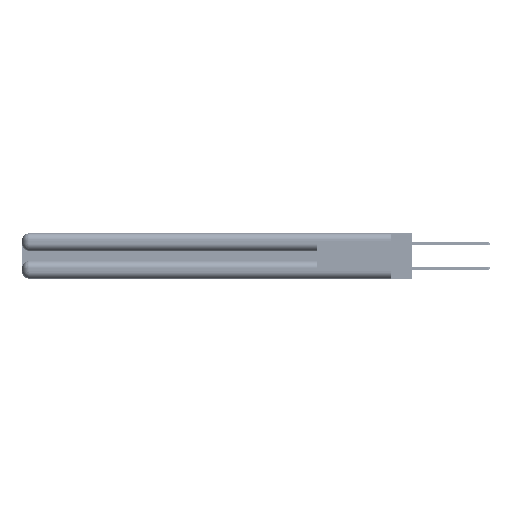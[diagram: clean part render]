
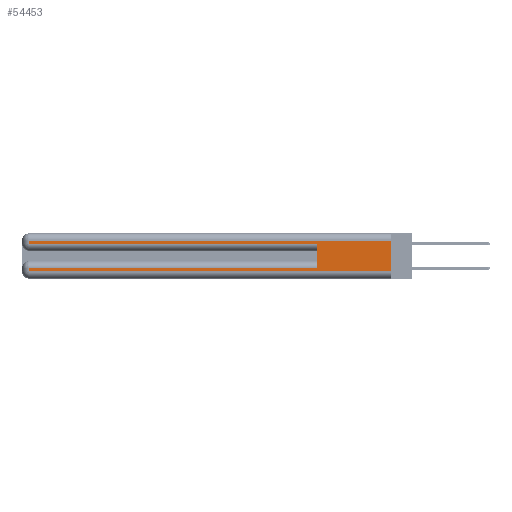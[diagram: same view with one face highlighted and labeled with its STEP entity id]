
A CAD part, left-side view. The second image highlights one B-rep face of the part: STEP entity #54453.
In plain terms, the highlighted planar face has unit normal (-1, 0, 0).
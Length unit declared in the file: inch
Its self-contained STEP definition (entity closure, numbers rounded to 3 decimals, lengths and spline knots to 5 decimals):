
#47 = ORIENTED_EDGE ( 'NONE', *, *, #4974, .T. ) ;
#947 = ORIENTED_EDGE ( 'NONE', *, *, #12364, .T. ) ;
#1749 = CARTESIAN_POINT ( 'NONE',  ( 0., 0.6, 0.285 ) ) ;
#1974 = VECTOR ( 'NONE', #44980, 39.37008 ) ;
#4145 = VECTOR ( 'NONE', #28373, 39.37008 ) ;
#4375 = DIRECTION ( 'NONE',  ( 0., 1., 0. ) ) ;
#4974 = EDGE_CURVE ( 'NONE', #36044, #13295, #21427, .T. ) ;
#5065 = VECTOR ( 'NONE', #9679, 39.37008 ) ;
#5963 = CARTESIAN_POINT ( 'NONE',  ( 0., 2.94, 0.085 ) ) ;
#7290 = ORIENTED_EDGE ( 'NONE', *, *, #31263, .F. ) ;
#8064 = VERTEX_POINT ( 'NONE', #47664 ) ;
#8731 = DIRECTION ( 'NONE',  ( 0., 0., -1. ) ) ;
#9679 = DIRECTION ( 'NONE',  ( 0., 0., -1. ) ) ;
#10702 = CARTESIAN_POINT ( 'NONE',  ( 0., 2.94, 0.285 ) ) ;
#10951 = DIRECTION ( 'NONE',  ( 0., -1., 0. ) ) ;
#12364 = EDGE_CURVE ( 'NONE', #24247, #8064, #53067, .T. ) ;
#13295 = VERTEX_POINT ( 'NONE', #27167 ) ;
#13397 = VERTEX_POINT ( 'NONE', #1749 ) ;
#13439 = EDGE_CURVE ( 'NONE', #8064, #55235, #55039, .T. ) ;
#14025 = CARTESIAN_POINT ( 'NONE',  ( 0., 0., 0.37 ) ) ;
#14072 = FACE_OUTER_BOUND ( 'NONE', #21732, .T. ) ;
#14508 = EDGE_CURVE ( 'NONE', #13295, #37177, #39589, .T. ) ;
#16024 = CARTESIAN_POINT ( 'NONE',  ( 0., 0., 0.37 ) ) ;
#16612 = EDGE_CURVE ( 'NONE', #40593, #13397, #27222, .T. ) ;
#17777 = EDGE_CURVE ( 'NONE', #37177, #13397, #35202, .T. ) ;
#18070 = VECTOR ( 'NONE', #20364, 39.37008 ) ;
#18396 = DIRECTION ( 'NONE',  ( 0., 0., -1. ) ) ;
#20364 = DIRECTION ( 'NONE',  ( 0., 0., -1. ) ) ;
#21288 = CARTESIAN_POINT ( 'NONE',  ( 0., 0.6, 0.085 ) ) ;
#21427 = LINE ( 'NONE', #52797, #44275 ) ;
#21708 = CARTESIAN_POINT ( 'NONE',  ( 0., 0., 0.085 ) ) ;
#21732 = EDGE_LOOP ( 'NONE', ( #7290, #47, #43941, #53854, #28434, #35657, #947, #35711 ) ) ;
#22550 = PLANE ( 'NONE',  #35473 ) ;
#22808 = DIRECTION ( 'NONE',  ( 0., 1., 0. ) ) ;
#24247 = VERTEX_POINT ( 'NONE', #5963 ) ;
#27167 = CARTESIAN_POINT ( 'NONE',  ( 0., 2.94, 0.31 ) ) ;
#27222 = LINE ( 'NONE', #41170, #4145 ) ;
#28373 = DIRECTION ( 'NONE',  ( 0., 0., 1. ) ) ;
#28434 = ORIENTED_EDGE ( 'NONE', *, *, #16612, .F. ) ;
#31263 = EDGE_CURVE ( 'NONE', #36044, #55235, #52309, .T. ) ;
#31639 = VECTOR ( 'NONE', #8731, 39.37008 ) ;
#35202 = LINE ( 'NONE', #44792, #1974 ) ;
#35473 = AXIS2_PLACEMENT_3D ( 'NONE', #14025, #44140, #18396 ) ;
#35657 = ORIENTED_EDGE ( 'NONE', *, *, #41909, .T. ) ;
#35711 = ORIENTED_EDGE ( 'NONE', *, *, #13439, .T. ) ;
#36044 = VERTEX_POINT ( 'NONE', #37216 ) ;
#37177 = VERTEX_POINT ( 'NONE', #10702 ) ;
#37216 = CARTESIAN_POINT ( 'NONE',  ( 0., 0., 0.31 ) ) ;
#39589 = LINE ( 'NONE', #39852, #5065 ) ;
#39852 = CARTESIAN_POINT ( 'NONE',  ( 0., 2.94, 0.37 ) ) ;
#40593 = VERTEX_POINT ( 'NONE', #21288 ) ;
#41093 = CARTESIAN_POINT ( 'NONE',  ( 0., 0., 0.06 ) ) ;
#41170 = CARTESIAN_POINT ( 'NONE',  ( 0., 0.6, 0.145 ) ) ;
#41909 = EDGE_CURVE ( 'NONE', #40593, #24247, #46632, .T. ) ;
#43736 = VECTOR ( 'NONE', #10951, 39.37008 ) ;
#43941 = ORIENTED_EDGE ( 'NONE', *, *, #14508, .T. ) ;
#44140 = DIRECTION ( 'NONE',  ( 1., 0., 0. ) ) ;
#44275 = VECTOR ( 'NONE', #22808, 39.37008 ) ;
#44792 = CARTESIAN_POINT ( 'NONE',  ( 0., 0., 0.285 ) ) ;
#44980 = DIRECTION ( 'NONE',  ( 0., -1., 0. ) ) ;
#45292 = VECTOR ( 'NONE', #4375, 39.37008 ) ;
#46632 = LINE ( 'NONE', #21708, #45292 ) ;
#47491 = CARTESIAN_POINT ( 'NONE',  ( 0., 2.94, 0.37 ) ) ;
#47664 = CARTESIAN_POINT ( 'NONE',  ( 0., 2.94, 0.06 ) ) ;
#50117 = CARTESIAN_POINT ( 'NONE',  ( 0., 0., 0.06 ) ) ;
#52309 = LINE ( 'NONE', #16024, #18070 ) ;
#52797 = CARTESIAN_POINT ( 'NONE',  ( 0., 0., 0.31 ) ) ;
#53067 = LINE ( 'NONE', #47491, #31639 ) ;
#53854 = ORIENTED_EDGE ( 'NONE', *, *, #17777, .T. ) ;
#54453 = ADVANCED_FACE ( 'NONE', ( #14072 ), #22550, .F. ) ;
#55039 = LINE ( 'NONE', #41093, #43736 ) ;
#55235 = VERTEX_POINT ( 'NONE', #50117 ) ;
